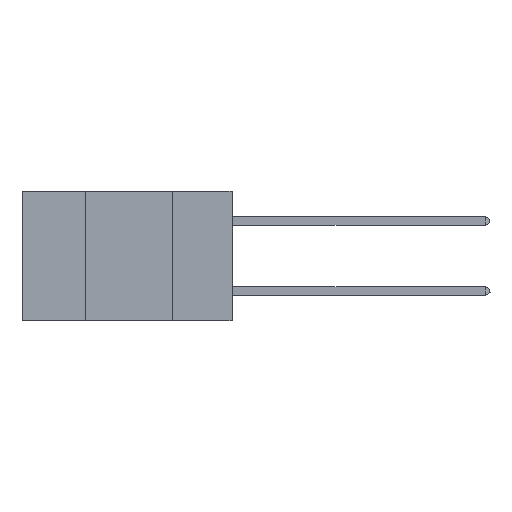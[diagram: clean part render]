
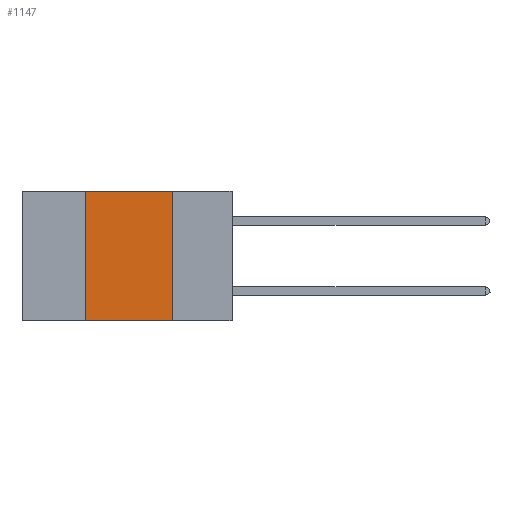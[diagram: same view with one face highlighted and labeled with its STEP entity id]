
A CAD part, left-side view. The second image highlights one B-rep face of the part: STEP entity #1147.
In plain terms, the highlighted planar face has unit normal (-1, 0, 0).
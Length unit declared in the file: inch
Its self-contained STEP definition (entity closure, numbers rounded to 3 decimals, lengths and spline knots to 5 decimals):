
#492 = EDGE_CURVE ( 'NONE', #9832, #10161, #2278, .T. ) ;
#1147 = ADVANCED_FACE ( 'NONE', ( #3270 ), #15129, .F. ) ;
#1968 = DIRECTION ( 'NONE',  ( 0., -1., 0. ) ) ;
#2230 = DIRECTION ( 'NONE',  ( 0., 0., 1. ) ) ;
#2278 = LINE ( 'NONE', #4826, #11660 ) ;
#3270 = FACE_OUTER_BOUND ( 'NONE', #5739, .T. ) ;
#3862 = LINE ( 'NONE', #14136, #8838 ) ;
#4354 = EDGE_CURVE ( 'NONE', #5665, #9832, #13807, .T. ) ;
#4784 = VECTOR ( 'NONE', #1968, 39.37008 ) ;
#4826 = CARTESIAN_POINT ( 'NONE',  ( 0., 0.17, 0. ) ) ;
#5416 = ORIENTED_EDGE ( 'NONE', *, *, #4354, .F. ) ;
#5665 = VERTEX_POINT ( 'NONE', #7253 ) ;
#5739 = EDGE_LOOP ( 'NONE', ( #9281, #5416, #12570, #11006 ) ) ;
#6404 = DIRECTION ( 'NONE',  ( 0., -1., 0. ) ) ;
#6523 = CARTESIAN_POINT ( 'NONE',  ( 0., 0.6, 0. ) ) ;
#7253 = CARTESIAN_POINT ( 'NONE',  ( 0., 0.42, 0. ) ) ;
#8377 = CARTESIAN_POINT ( 'NONE',  ( 0., 0.17, 0. ) ) ;
#8838 = VECTOR ( 'NONE', #6404, 39.37008 ) ;
#9281 = ORIENTED_EDGE ( 'NONE', *, *, #492, .F. ) ;
#9832 = VERTEX_POINT ( 'NONE', #8377 ) ;
#9842 = CARTESIAN_POINT ( 'NONE',  ( 0., 0.42, 0. ) ) ;
#10147 = DIRECTION ( 'NONE',  ( 0., 0., -1. ) ) ;
#10161 = VERTEX_POINT ( 'NONE', #10884 ) ;
#10884 = CARTESIAN_POINT ( 'NONE',  ( 0., 0.17, -0.37 ) ) ;
#11006 = ORIENTED_EDGE ( 'NONE', *, *, #12480, .T. ) ;
#11645 = DIRECTION ( 'NONE',  ( 1., 0., 0. ) ) ;
#11660 = VECTOR ( 'NONE', #16306, 39.37008 ) ;
#12311 = VECTOR ( 'NONE', #2230, 39.37008 ) ;
#12480 = EDGE_CURVE ( 'NONE', #12494, #10161, #3862, .T. ) ;
#12494 = VERTEX_POINT ( 'NONE', #14235 ) ;
#12570 = ORIENTED_EDGE ( 'NONE', *, *, #12626, .F. ) ;
#12626 = EDGE_CURVE ( 'NONE', #12494, #5665, #15721, .T. ) ;
#13320 = AXIS2_PLACEMENT_3D ( 'NONE', #6523, #11645, #10147 ) ;
#13807 = LINE ( 'NONE', #14708, #4784 ) ;
#14136 = CARTESIAN_POINT ( 'NONE',  ( 0., 0.6, -0.37 ) ) ;
#14235 = CARTESIAN_POINT ( 'NONE',  ( 0., 0.42, -0.37 ) ) ;
#14708 = CARTESIAN_POINT ( 'NONE',  ( 0., 0.6, 0. ) ) ;
#15129 = PLANE ( 'NONE',  #13320 ) ;
#15721 = LINE ( 'NONE', #9842, #12311 ) ;
#16306 = DIRECTION ( 'NONE',  ( 0., 0., -1. ) ) ;
